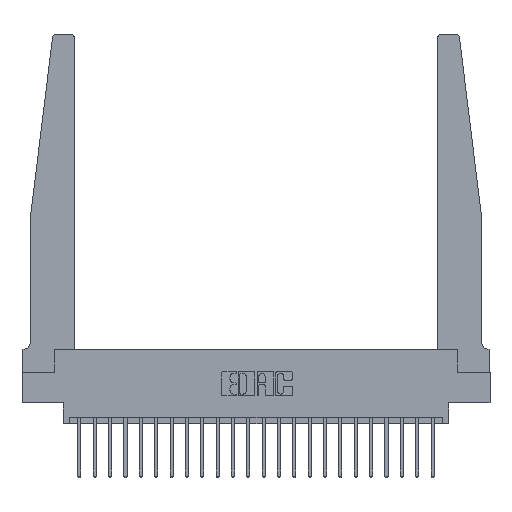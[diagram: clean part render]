
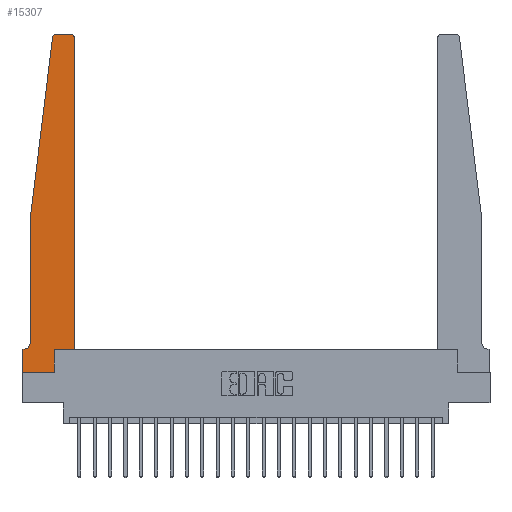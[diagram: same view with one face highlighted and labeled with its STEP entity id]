
A CAD part, top view. The second image highlights one B-rep face of the part: STEP entity #15307.
In plain terms, the highlighted planar face has unit normal (0, 0, 1).
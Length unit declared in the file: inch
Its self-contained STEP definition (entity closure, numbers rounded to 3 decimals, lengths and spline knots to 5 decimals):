
#91 = EDGE_CURVE ( 'NONE', #18297, #23280, #8899, .T. ) ;
#1434 = DIRECTION ( 'NONE',  ( -1., 0., 0. ) ) ;
#1471 = LINE ( 'NONE', #15734, #21559 ) ;
#1575 = EDGE_CURVE ( 'NONE', #19443, #23276, #1471, .T. ) ;
#2063 = ORIENTED_EDGE ( 'NONE', *, *, #17748, .T. ) ;
#2537 = ORIENTED_EDGE ( 'NONE', *, *, #22704, .T. ) ;
#2661 = VECTOR ( 'NONE', #11058, 39.37008 ) ;
#3564 = CARTESIAN_POINT ( 'NONE',  ( 0.425, 0.18, 0.37 ) ) ;
#3995 = CARTESIAN_POINT ( 'NONE',  ( 0.425, 0.18, 0.37 ) ) ;
#4275 = VECTOR ( 'NONE', #15811, 39.37008 ) ;
#4912 = CIRCLE ( 'NONE', #10605, 0.03 ) ;
#5002 = CARTESIAN_POINT ( 'NONE',  ( 0.425, 2.72, 0.37 ) ) ;
#5635 = VECTOR ( 'NONE', #11222, 39.37008 ) ;
#6337 = DIRECTION ( 'NONE',  ( -0.122, -0.992, 0. ) ) ;
#6509 = DIRECTION ( 'NONE',  ( 0., 0., 1. ) ) ;
#6543 = DIRECTION ( 'NONE',  ( 0., -1., 0. ) ) ;
#6653 = LINE ( 'NONE', #11763, #7686 ) ;
#6781 = CARTESIAN_POINT ( 'NONE',  ( 0.065, 0.2375, 0.37 ) ) ;
#6901 = CARTESIAN_POINT ( 'NONE',  ( 0.395, 2.72, 0.37 ) ) ;
#7038 = CARTESIAN_POINT ( 'NONE',  ( 0.015, 0.2375, 0.37 ) ) ;
#7330 = AXIS2_PLACEMENT_3D ( 'NONE', #7038, #10822, #1434 ) ;
#7535 = EDGE_CURVE ( 'NONE', #13363, #18297, #22269, .T. ) ;
#7578 = VECTOR ( 'NONE', #10032, 39.37008 ) ;
#7601 = VERTEX_POINT ( 'NONE', #12139 ) ;
#7628 = CARTESIAN_POINT ( 'NONE',  ( 0.395, 2.75, 0.37 ) ) ;
#7686 = VECTOR ( 'NONE', #6543, 39.37008 ) ;
#7709 = EDGE_CURVE ( 'NONE', #7601, #13363, #10827, .T. ) ;
#7933 = CARTESIAN_POINT ( 'NONE',  ( 0., 0.1875, 0.37 ) ) ;
#7967 = ORIENTED_EDGE ( 'NONE', *, *, #1575, .T. ) ;
#8045 = DIRECTION ( 'NONE',  ( 1., 0., 0. ) ) ;
#8093 = CARTESIAN_POINT ( 'NONE',  ( 0., 0., 0.37 ) ) ;
#8288 = ORIENTED_EDGE ( 'NONE', *, *, #13771, .T. ) ;
#8667 = ORIENTED_EDGE ( 'NONE', *, *, #22196, .T. ) ;
#8899 = LINE ( 'NONE', #10910, #20209 ) ;
#9195 = VECTOR ( 'NONE', #15970, 39.37008 ) ;
#10032 = DIRECTION ( 'NONE',  ( -1., 0., 0. ) ) ;
#10054 = CARTESIAN_POINT ( 'NONE',  ( 0., 0.1875, 0.37 ) ) ;
#10087 = VERTEX_POINT ( 'NONE', #18735 ) ;
#10170 = VERTEX_POINT ( 'NONE', #10054 ) ;
#10605 = AXIS2_PLACEMENT_3D ( 'NONE', #6901, #19600, #12596 ) ;
#10822 = DIRECTION ( 'NONE',  ( 0., 0., -1. ) ) ;
#10827 = LINE ( 'NONE', #14736, #2661 ) ;
#10910 = CARTESIAN_POINT ( 'NONE',  ( 0.425, 0.18, 0.37 ) ) ;
#11058 = DIRECTION ( 'NONE',  ( 0., 1., 0. ) ) ;
#11222 = DIRECTION ( 'NONE',  ( 1., 0., 0. ) ) ;
#11257 = PLANE ( 'NONE',  #17485 ) ;
#11763 = CARTESIAN_POINT ( 'NONE',  ( 0., 0., 0.37 ) ) ;
#11856 = CARTESIAN_POINT ( 'NONE',  ( 0.27653, 2.72, 0.37 ) ) ;
#12062 = ORIENTED_EDGE ( 'NONE', *, *, #17919, .T. ) ;
#12139 = CARTESIAN_POINT ( 'NONE',  ( 0.2605, 0., 0.37 ) ) ;
#12227 = CIRCLE ( 'NONE', #7330, 0.05 ) ;
#12312 = ORIENTED_EDGE ( 'NONE', *, *, #15950, .T. ) ;
#12596 = DIRECTION ( 'NONE',  ( 1., 0., 0. ) ) ;
#12958 = DIRECTION ( 'NONE',  ( 1., 0., 0. ) ) ;
#12993 = EDGE_CURVE ( 'NONE', #10087, #16998, #17145, .T. ) ;
#13363 = VERTEX_POINT ( 'NONE', #15593 ) ;
#13600 = CARTESIAN_POINT ( 'NONE',  ( 0.25, 2.75, 0.37 ) ) ;
#13671 = CARTESIAN_POINT ( 'NONE',  ( 0.065, 1.25, 0.37 ) ) ;
#13771 = EDGE_CURVE ( 'NONE', #10170, #21463, #6653, .T. ) ;
#14736 = CARTESIAN_POINT ( 'NONE',  ( 0.2605, 0.18, 0.37 ) ) ;
#14868 = AXIS2_PLACEMENT_3D ( 'NONE', #11856, #6509, #8045 ) ;
#14893 = VERTEX_POINT ( 'NONE', #16564 ) ;
#15307 = ADVANCED_FACE ( 'NONE', ( #18413 ), #11257, .T. ) ;
#15593 = CARTESIAN_POINT ( 'NONE',  ( 0.2605, 0.18, 0.37 ) ) ;
#15734 = CARTESIAN_POINT ( 'NONE',  ( 0.065, 1.25, 0.37 ) ) ;
#15811 = DIRECTION ( 'NONE',  ( 1., 0., 0. ) ) ;
#15950 = EDGE_CURVE ( 'NONE', #16998, #19443, #19062, .T. ) ;
#15970 = DIRECTION ( 'NONE',  ( -1., 0., 0. ) ) ;
#16163 = VERTEX_POINT ( 'NONE', #7628 ) ;
#16564 = CARTESIAN_POINT ( 'NONE',  ( 0.015, 0.1875, 0.37 ) ) ;
#16734 = VECTOR ( 'NONE', #6337, 39.37008 ) ;
#16761 = EDGE_LOOP ( 'NONE', ( #22817, #19729, #12312, #7967, #12062, #2537, #8288, #2063, #19133, #22285, #20994, #8667 ) ) ;
#16998 = VERTEX_POINT ( 'NONE', #18017 ) ;
#17018 = LINE ( 'NONE', #22375, #7578 ) ;
#17145 = CIRCLE ( 'NONE', #14868, 0.03 ) ;
#17259 = EDGE_CURVE ( 'NONE', #16163, #10087, #17635, .T. ) ;
#17485 = AXIS2_PLACEMENT_3D ( 'NONE', #7933, #21861, #12958 ) ;
#17635 = LINE ( 'NONE', #13600, #9195 ) ;
#17748 = EDGE_CURVE ( 'NONE', #21463, #7601, #19507, .T. ) ;
#17919 = EDGE_CURVE ( 'NONE', #23276, #14893, #12227, .T. ) ;
#18017 = CARTESIAN_POINT ( 'NONE',  ( 0.24675, 2.72367, 0.37 ) ) ;
#18159 = DIRECTION ( 'NONE',  ( 0., 1., 0. ) ) ;
#18297 = VERTEX_POINT ( 'NONE', #3564 ) ;
#18413 = FACE_OUTER_BOUND ( 'NONE', #16761, .T. ) ;
#18735 = CARTESIAN_POINT ( 'NONE',  ( 0.27653, 2.75, 0.37 ) ) ;
#19062 = LINE ( 'NONE', #22618, #16734 ) ;
#19133 = ORIENTED_EDGE ( 'NONE', *, *, #7709, .T. ) ;
#19443 = VERTEX_POINT ( 'NONE', #13671 ) ;
#19507 = LINE ( 'NONE', #8093, #4275 ) ;
#19600 = DIRECTION ( 'NONE',  ( 0., 0., 1. ) ) ;
#19729 = ORIENTED_EDGE ( 'NONE', *, *, #12993, .T. ) ;
#20209 = VECTOR ( 'NONE', #18159, 39.37008 ) ;
#20994 = ORIENTED_EDGE ( 'NONE', *, *, #91, .T. ) ;
#21463 = VERTEX_POINT ( 'NONE', #22492 ) ;
#21559 = VECTOR ( 'NONE', #23204, 39.37008 ) ;
#21861 = DIRECTION ( 'NONE',  ( 0., 0., 1. ) ) ;
#22196 = EDGE_CURVE ( 'NONE', #23280, #16163, #4912, .T. ) ;
#22269 = LINE ( 'NONE', #3995, #5635 ) ;
#22285 = ORIENTED_EDGE ( 'NONE', *, *, #7535, .T. ) ;
#22375 = CARTESIAN_POINT ( 'NONE',  ( 0.065, 0.1875, 0.37 ) ) ;
#22492 = CARTESIAN_POINT ( 'NONE',  ( 0., 0., 0.37 ) ) ;
#22618 = CARTESIAN_POINT ( 'NONE',  ( 0.065, 1.25, 0.37 ) ) ;
#22704 = EDGE_CURVE ( 'NONE', #14893, #10170, #17018, .T. ) ;
#22817 = ORIENTED_EDGE ( 'NONE', *, *, #17259, .T. ) ;
#23204 = DIRECTION ( 'NONE',  ( 0., -1., 0. ) ) ;
#23276 = VERTEX_POINT ( 'NONE', #6781 ) ;
#23280 = VERTEX_POINT ( 'NONE', #5002 ) ;
